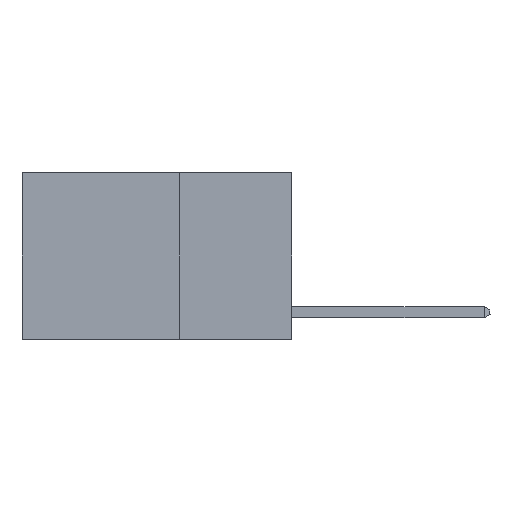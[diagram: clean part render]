
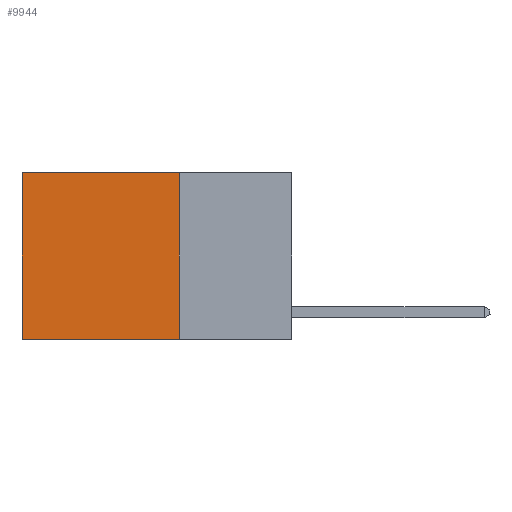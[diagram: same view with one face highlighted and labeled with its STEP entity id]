
A CAD part, left-side view. The second image highlights one B-rep face of the part: STEP entity #9944.
In plain terms, the highlighted planar face has unit normal (-1, 0, 0).
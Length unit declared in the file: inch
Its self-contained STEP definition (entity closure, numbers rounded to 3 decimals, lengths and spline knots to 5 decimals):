
#697 = CARTESIAN_POINT ( 'NONE',  ( 0.2625, 0.25, 0. ) ) ;
#1216 = CARTESIAN_POINT ( 'NONE',  ( 0.2625, 0.25, 0. ) ) ;
#1683 = CARTESIAN_POINT ( 'NONE',  ( 0.2625, 0.6, 0. ) ) ;
#2710 = CARTESIAN_POINT ( 'NONE',  ( 0.2625, 0.25, 0. ) ) ;
#2764 = VERTEX_POINT ( 'NONE', #1683 ) ;
#3955 = ORIENTED_EDGE ( 'NONE', *, *, #10230, .F. ) ;
#3976 = VERTEX_POINT ( 'NONE', #7961 ) ;
#4387 = VECTOR ( 'NONE', #5503, 39.37008 ) ;
#4538 = EDGE_CURVE ( 'NONE', #6878, #2764, #26325, .T. ) ;
#5503 = DIRECTION ( 'NONE',  ( 0., 1., 0. ) ) ;
#5602 = EDGE_LOOP ( 'NONE', ( #16942, #3955, #9143, #18279 ) ) ;
#6878 = VERTEX_POINT ( 'NONE', #697 ) ;
#7782 = PLANE ( 'NONE',  #12561 ) ;
#7961 = CARTESIAN_POINT ( 'NONE',  ( 0.2625, 0.6, -0.37 ) ) ;
#8141 = EDGE_CURVE ( 'NONE', #6878, #22634, #12904, .T. ) ;
#8450 = VECTOR ( 'NONE', #20768, 39.37008 ) ;
#8802 = CARTESIAN_POINT ( 'NONE',  ( 0.2625, 0.25, -0.37 ) ) ;
#9143 = ORIENTED_EDGE ( 'NONE', *, *, #8141, .F. ) ;
#9944 = ADVANCED_FACE ( 'NONE', ( #12134 ), #7782, .F. ) ;
#9957 = DIRECTION ( 'NONE',  ( 1., 0., 0. ) ) ;
#10230 = EDGE_CURVE ( 'NONE', #22634, #3976, #14748, .T. ) ;
#10932 = DIRECTION ( 'NONE',  ( 0., 1., 0. ) ) ;
#12134 = FACE_OUTER_BOUND ( 'NONE', #5602, .T. ) ;
#12561 = AXIS2_PLACEMENT_3D ( 'NONE', #18369, #9957, #24818 ) ;
#12904 = LINE ( 'NONE', #2710, #18517 ) ;
#13343 = DIRECTION ( 'NONE',  ( 0., 0., -1. ) ) ;
#14748 = LINE ( 'NONE', #8802, #25409 ) ;
#14786 = CARTESIAN_POINT ( 'NONE',  ( 0.2625, 0.25, -0.37 ) ) ;
#15410 = EDGE_CURVE ( 'NONE', #2764, #3976, #25429, .T. ) ;
#16942 = ORIENTED_EDGE ( 'NONE', *, *, #15410, .T. ) ;
#18279 = ORIENTED_EDGE ( 'NONE', *, *, #4538, .T. ) ;
#18369 = CARTESIAN_POINT ( 'NONE',  ( 0.2625, 0.25, 0. ) ) ;
#18517 = VECTOR ( 'NONE', #13343, 39.37008 ) ;
#18632 = CARTESIAN_POINT ( 'NONE',  ( 0.2625, 0.6, 0. ) ) ;
#20768 = DIRECTION ( 'NONE',  ( 0., 0., -1. ) ) ;
#22634 = VERTEX_POINT ( 'NONE', #14786 ) ;
#24818 = DIRECTION ( 'NONE',  ( 0., 0., -1. ) ) ;
#25409 = VECTOR ( 'NONE', #10932, 39.37008 ) ;
#25429 = LINE ( 'NONE', #18632, #8450 ) ;
#26325 = LINE ( 'NONE', #1216, #4387 ) ;
